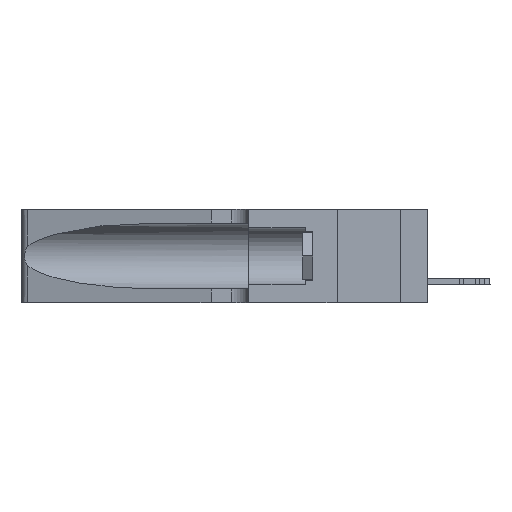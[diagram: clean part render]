
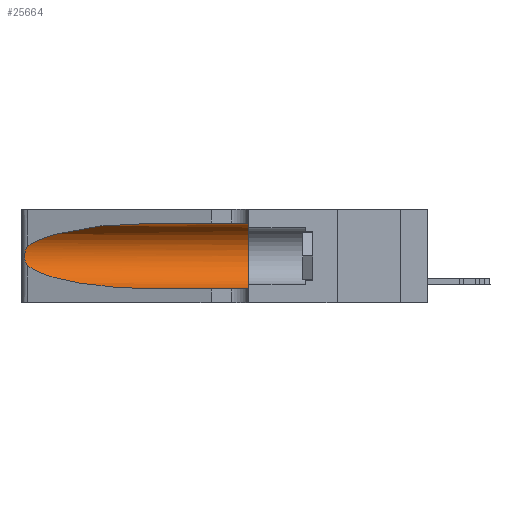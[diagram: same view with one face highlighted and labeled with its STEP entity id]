
A CAD part, left-side view. The second image highlights one B-rep face of the part: STEP entity #25664.
In plain terms, the highlighted cylindrical face has radius 3.308 mm (diameter 6.617 mm), a partial arc.
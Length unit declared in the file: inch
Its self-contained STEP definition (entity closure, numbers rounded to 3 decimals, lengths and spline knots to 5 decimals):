
#1008 = CARTESIAN_POINT ( 'NONE',  ( 0.25854, 1.2359, 0.20912 ) ) ;
#1028 = ORIENTED_EDGE ( 'NONE', *, *, #2739, .T. ) ;
#1096 = AXIS2_PLACEMENT_3D ( 'NONE', #31414, #20983, #4322 ) ;
#1273 = VECTOR ( 'NONE', #13873, 39.37008 ) ;
#1489 = VERTEX_POINT ( 'NONE', #41486 ) ;
#2491 = CARTESIAN_POINT ( 'NONE',  ( 0.25555, 1.22994, 0.2215 ) ) ;
#2624 =( BOUNDED_CURVE ( )  B_SPLINE_CURVE ( 3, ( #42301, #13645, #23115, #39675 ),
 .UNSPECIFIED., .F., .F. ) 
 B_SPLINE_CURVE_WITH_KNOTS ( ( 4, 4 ),
 ( 3.44316, 4.71239 ),
 .UNSPECIFIED. ) 
 CURVE ( )  GEOMETRIC_REPRESENTATION_ITEM ( )  RATIONAL_B_SPLINE_CURVE ( ( 1., 0.87, 0.87, 1. ) ) 
 REPRESENTATION_ITEM ( '' )  );
#2739 = EDGE_CURVE ( 'NONE', #28248, #9672, #37303, .T. ) ;
#3548 = CYLINDRICAL_SURFACE ( 'NONE', #29005, 0.13025 ) ;
#3823 = EDGE_CURVE ( 'NONE', #28248, #41916, #21207, .T. ) ;
#3991 = CARTESIAN_POINT ( 'NONE',  ( 0.2373, 1.15595, 0.28018 ) ) ;
#4245 = ORIENTED_EDGE ( 'NONE', *, *, #33249, .T. ) ;
#4322 = DIRECTION ( 'NONE',  ( 0., 0., 1. ) ) ;
#4367 = VERTEX_POINT ( 'NONE', #8594 ) ;
#5780 = EDGE_CURVE ( 'NONE', #9672, #1489, #42653, .T. ) ;
#6234 = CARTESIAN_POINT ( 'NONE',  ( 0.1305, 1.61858, 0.185 ) ) ;
#7322 = CARTESIAN_POINT ( 'NONE',  ( 0.25487, 1.22718, 0.22369 ) ) ;
#8594 = CARTESIAN_POINT ( 'NONE',  ( 0.1305, 0.35, 0.05475 ) ) ;
#9672 = VERTEX_POINT ( 'NONE', #11362 ) ;
#9917 = DIRECTION ( 'NONE',  ( 0., 0., -1. ) ) ;
#11362 = CARTESIAN_POINT ( 'NONE',  ( 0.25487, 1.22718, 0.22369 ) ) ;
#12573 = EDGE_CURVE ( 'NONE', #41916, #4367, #41915, .T. ) ;
#13170 = CARTESIAN_POINT ( 'NONE',  ( 0.1305, 1.61858, 0.31525 ) ) ;
#13645 = CARTESIAN_POINT ( 'NONE',  ( 0.2373, 1.15595, 0.08982 ) ) ;
#13873 = DIRECTION ( 'NONE',  ( 0., -1., 0. ) ) ;
#15342 = CARTESIAN_POINT ( 'NONE',  ( 0.25639, 1.23186, 0.15144 ) ) ;
#16512 = CARTESIAN_POINT ( 'NONE',  ( 0.25487, 1.22718, 0.22369 ) ) ;
#16618 = CARTESIAN_POINT ( 'NONE',  ( 0.26075, 1.23896, 0.178 ) ) ;
#16796 = VERTEX_POINT ( 'NONE', #32315 ) ;
#17051 = ORIENTED_EDGE ( 'NONE', *, *, #37833, .T. ) ;
#17643 = CARTESIAN_POINT ( 'NONE',  ( 0.1305, 1.61858, 0.05475 ) ) ;
#18856 = EDGE_LOOP ( 'NONE', ( #1028, #37836, #4245, #17051, #29834, #33086 ) ) ;
#19252 = CARTESIAN_POINT ( 'NONE',  ( 0.25789, 1.23486, 0.15765 ) ) ;
#20983 = DIRECTION ( 'NONE',  ( 0., 1., 0. ) ) ;
#21099 = LINE ( 'NONE', #17643, #1273 ) ;
#21207 = LINE ( 'NONE', #13170, #30536 ) ;
#23115 = CARTESIAN_POINT ( 'NONE',  ( 0.18966, 0.96281, 0.05475 ) ) ;
#25480 = FACE_OUTER_BOUND ( 'NONE', #18856, .T. ) ;
#25664 = ADVANCED_FACE ( 'NONE', ( #25480 ), #3548, .F. ) ;
#25797 = CARTESIAN_POINT ( 'NONE',  ( 0.25639, 1.23184, 0.21858 ) ) ;
#28248 = VERTEX_POINT ( 'NONE', #38905 ) ;
#29005 = AXIS2_PLACEMENT_3D ( 'NONE', #6234, #40004, #9917 ) ;
#29141 = CARTESIAN_POINT ( 'NONE',  ( 0.25787, 1.23484, 0.2124 ) ) ;
#29834 = ORIENTED_EDGE ( 'NONE', *, *, #12573, .F. ) ;
#30536 = VECTOR ( 'NONE', #39460, 39.37008 ) ;
#30774 = CARTESIAN_POINT ( 'NONE',  ( 0.18966, 0.96281, 0.31525 ) ) ;
#31200 = CARTESIAN_POINT ( 'NONE',  ( 0.1305, 0.72297, 0.31525 ) ) ;
#31226 = CARTESIAN_POINT ( 'NONE',  ( 0.1305, 0.35, 0.31525 ) ) ;
#31414 = CARTESIAN_POINT ( 'NONE',  ( 0.1305, 0.35, 0.185 ) ) ;
#32315 = CARTESIAN_POINT ( 'NONE',  ( 0.1305, 0.72297, 0.05475 ) ) ;
#33086 = ORIENTED_EDGE ( 'NONE', *, *, #3823, .F. ) ;
#33194 = CARTESIAN_POINT ( 'NONE',  ( 0.26075, 1.23896, 0.19203 ) ) ;
#33249 = EDGE_CURVE ( 'NONE', #1489, #16796, #2624, .T. ) ;
#36515 = CARTESIAN_POINT ( 'NONE',  ( 0.25856, 1.23593, 0.16098 ) ) ;
#37303 =( BOUNDED_CURVE ( )  B_SPLINE_CURVE ( 3, ( #31200, #30774, #3991, #7322 ),
 .UNSPECIFIED., .F., .F. ) 
 B_SPLINE_CURVE_WITH_KNOTS ( ( 4, 4 ),
 ( 1.5708, 2.84003 ),
 .UNSPECIFIED. ) 
 CURVE ( )  GEOMETRIC_REPRESENTATION_ITEM ( )  RATIONAL_B_SPLINE_CURVE ( ( 1., 0.87, 0.87, 1. ) ) 
 REPRESENTATION_ITEM ( '' )  );
#37833 = EDGE_CURVE ( 'NONE', #16796, #4367, #21099, .T. ) ;
#37836 = ORIENTED_EDGE ( 'NONE', *, *, #5780, .T. ) ;
#38276 = CARTESIAN_POINT ( 'NONE',  ( 0.25555, 1.22993, 0.14849 ) ) ;
#38423 = CARTESIAN_POINT ( 'NONE',  ( 0.25487, 1.22718, 0.14631 ) ) ;
#38905 = CARTESIAN_POINT ( 'NONE',  ( 0.1305, 0.72297, 0.31525 ) ) ;
#39460 = DIRECTION ( 'NONE',  ( 0., -1., 0. ) ) ;
#39675 = CARTESIAN_POINT ( 'NONE',  ( 0.1305, 0.72297, 0.05475 ) ) ;
#39696 = CARTESIAN_POINT ( 'NONE',  ( 0.26017, 1.23833, 0.17102 ) ) ;
#40004 = DIRECTION ( 'NONE',  ( 0., -1., 0. ) ) ;
#41003 = CARTESIAN_POINT ( 'NONE',  ( 0.26018, 1.23835, 0.19895 ) ) ;
#41486 = CARTESIAN_POINT ( 'NONE',  ( 0.25487, 1.22718, 0.14631 ) ) ;
#41915 = CIRCLE ( 'NONE', #1096, 0.13025 ) ;
#41916 = VERTEX_POINT ( 'NONE', #31226 ) ;
#42301 = CARTESIAN_POINT ( 'NONE',  ( 0.25487, 1.22718, 0.14631 ) ) ;
#42653 = B_SPLINE_CURVE_WITH_KNOTS ( 'NONE', 3,
 ( #16512, #2491, #25797, #29141, #1008, #41003, #33194, #16618, #39696, #36515, #19252, #15342, #38276, #38423 ),
 .UNSPECIFIED., .F., .F.,
 ( 4, 2, 2, 2, 2, 2, 4 ),
 ( 0., 0.00027, 0.00053, 0.00107, 0.0016, 0.00187, 0.00214 ),
 .UNSPECIFIED. ) ;
